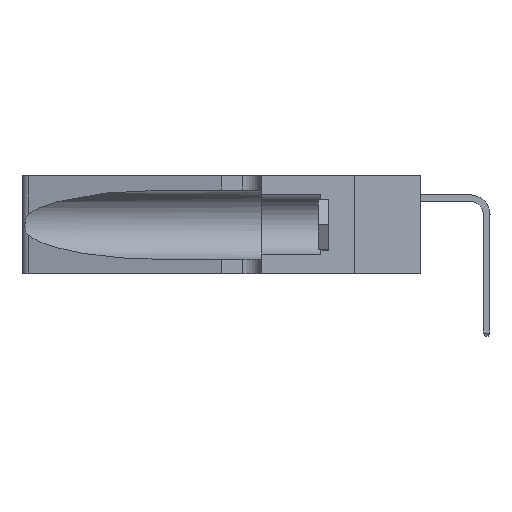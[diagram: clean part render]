
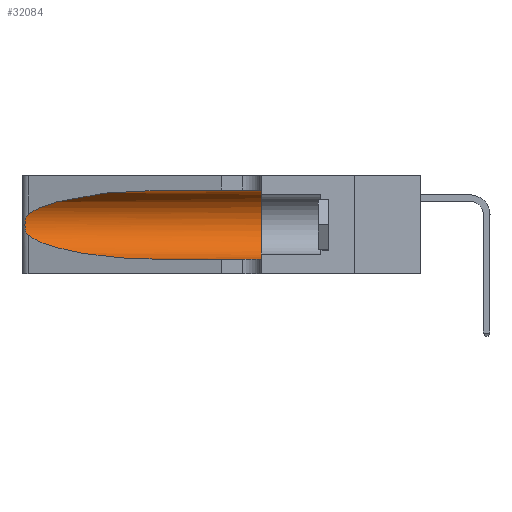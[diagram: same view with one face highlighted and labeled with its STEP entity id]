
A CAD part, left-side view. The second image highlights one B-rep face of the part: STEP entity #32084.
In plain terms, the highlighted cylindrical face has radius 3.308 mm (diameter 6.617 mm), a partial arc.
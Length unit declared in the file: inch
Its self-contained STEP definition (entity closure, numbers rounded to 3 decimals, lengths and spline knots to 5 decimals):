
#2858 = LINE ( 'NONE', #45929, #22922 ) ;
#3886 = CARTESIAN_POINT ( 'NONE',  ( 0.25787, 1.23484, 0.2124 ) ) ;
#4280 = ORIENTED_EDGE ( 'NONE', *, *, #10704, .T. ) ;
#4715 = CARTESIAN_POINT ( 'NONE',  ( 0.1305, 0.35, 0.05475 ) ) ;
#7629 = CARTESIAN_POINT ( 'NONE',  ( 0.26018, 1.23835, 0.19895 ) ) ;
#7790 = LINE ( 'NONE', #32172, #27895 ) ;
#8375 =( BOUNDED_CURVE ( )  B_SPLINE_CURVE ( 3, ( #46101, #42348, #19927, #23691 ),
 .UNSPECIFIED., .F., .F. ) 
 B_SPLINE_CURVE_WITH_KNOTS ( ( 4, 4 ),
 ( 1.5708, 2.84003 ),
 .UNSPECIFIED. ) 
 CURVE ( )  GEOMETRIC_REPRESENTATION_ITEM ( )  RATIONAL_B_SPLINE_CURVE ( ( 1., 0.87, 0.87, 1. ) ) 
 REPRESENTATION_ITEM ( '' )  );
#9575 = DIRECTION ( 'NONE',  ( 0., -1., 0. ) ) ;
#10704 = EDGE_CURVE ( 'NONE', #14904, #12338, #38522, .T. ) ;
#11465 = CARTESIAN_POINT ( 'NONE',  ( 0.26075, 1.23896, 0.178 ) ) ;
#12136 = EDGE_CURVE ( 'NONE', #32609, #28590, #2858, .T. ) ;
#12164 = EDGE_CURVE ( 'NONE', #32609, #22208, #8375, .T. ) ;
#12338 = VERTEX_POINT ( 'NONE', #47231 ) ;
#13855 = B_SPLINE_CURVE_WITH_KNOTS ( 'NONE', 3,
 ( #45111, #18906, #26467, #3886, #30233, #7629, #33977, #11465, #37732, #15300, #41510, #19059, #45274, #22856 ),
 .UNSPECIFIED., .F., .F.,
 ( 4, 2, 2, 2, 2, 2, 4 ),
 ( 0., 0.00027, 0.00053, 0.00107, 0.0016, 0.00187, 0.00214 ),
 .UNSPECIFIED. ) ;
#13954 = DIRECTION ( 'NONE',  ( 0., 0., -1. ) ) ;
#14749 = CARTESIAN_POINT ( 'NONE',  ( 0.18966, 0.96281, 0.05475 ) ) ;
#14904 = VERTEX_POINT ( 'NONE', #39498 ) ;
#15300 = CARTESIAN_POINT ( 'NONE',  ( 0.25856, 1.23593, 0.16098 ) ) ;
#16971 = EDGE_CURVE ( 'NONE', #28590, #46605, #36760, .T. ) ;
#18906 = CARTESIAN_POINT ( 'NONE',  ( 0.25555, 1.22994, 0.2215 ) ) ;
#19059 = CARTESIAN_POINT ( 'NONE',  ( 0.25639, 1.23186, 0.15144 ) ) ;
#19927 = CARTESIAN_POINT ( 'NONE',  ( 0.2373, 1.15595, 0.28018 ) ) ;
#21382 = CARTESIAN_POINT ( 'NONE',  ( 0.1305, 0.35, 0.31525 ) ) ;
#21404 = DIRECTION ( 'NONE',  ( 0., 1., 0. ) ) ;
#22028 = CYLINDRICAL_SURFACE ( 'NONE', #26844, 0.13025 ) ;
#22208 = VERTEX_POINT ( 'NONE', #44135 ) ;
#22330 = CARTESIAN_POINT ( 'NONE',  ( 0.25487, 1.22718, 0.14631 ) ) ;
#22856 = CARTESIAN_POINT ( 'NONE',  ( 0.25487, 1.22718, 0.14631 ) ) ;
#22922 = VECTOR ( 'NONE', #38398, 39.37008 ) ;
#23357 = ORIENTED_EDGE ( 'NONE', *, *, #12136, .F. ) ;
#23691 = CARTESIAN_POINT ( 'NONE',  ( 0.25487, 1.22718, 0.22369 ) ) ;
#26467 = CARTESIAN_POINT ( 'NONE',  ( 0.25639, 1.23184, 0.21858 ) ) ;
#26844 = AXIS2_PLACEMENT_3D ( 'NONE', #28940, #40171, #13954 ) ;
#26999 = ORIENTED_EDGE ( 'NONE', *, *, #12164, .T. ) ;
#27895 = VECTOR ( 'NONE', #9575, 39.37008 ) ;
#28590 = VERTEX_POINT ( 'NONE', #21382 ) ;
#28940 = CARTESIAN_POINT ( 'NONE',  ( 0.1305, 1.61858, 0.185 ) ) ;
#30233 = CARTESIAN_POINT ( 'NONE',  ( 0.25854, 1.2359, 0.20912 ) ) ;
#32084 = ADVANCED_FACE ( 'NONE', ( #41922 ), #22028, .F. ) ;
#32172 = CARTESIAN_POINT ( 'NONE',  ( 0.1305, 1.61858, 0.05475 ) ) ;
#32609 = VERTEX_POINT ( 'NONE', #36390 ) ;
#32693 = EDGE_LOOP ( 'NONE', ( #26999, #33286, #4280, #45901, #33306, #23357 ) ) ;
#33286 = ORIENTED_EDGE ( 'NONE', *, *, #44999, .T. ) ;
#33306 = ORIENTED_EDGE ( 'NONE', *, *, #16971, .F. ) ;
#33977 = CARTESIAN_POINT ( 'NONE',  ( 0.26075, 1.23896, 0.19203 ) ) ;
#36145 = AXIS2_PLACEMENT_3D ( 'NONE', #43827, #21404, #47603 ) ;
#36390 = CARTESIAN_POINT ( 'NONE',  ( 0.1305, 0.72297, 0.31525 ) ) ;
#36760 = CIRCLE ( 'NONE', #36145, 0.13025 ) ;
#37732 = CARTESIAN_POINT ( 'NONE',  ( 0.26017, 1.23833, 0.17102 ) ) ;
#38398 = DIRECTION ( 'NONE',  ( 0., -1., 0. ) ) ;
#38522 =( BOUNDED_CURVE ( )  B_SPLINE_CURVE ( 3, ( #22330, #40964, #14749, #48524 ),
 .UNSPECIFIED., .F., .T. ) 
 B_SPLINE_CURVE_WITH_KNOTS ( ( 4, 4 ),
 ( 3.44316, 4.71239 ),
 .UNSPECIFIED. ) 
 CURVE ( )  GEOMETRIC_REPRESENTATION_ITEM ( )  RATIONAL_B_SPLINE_CURVE ( ( 1., 0.87, 0.87, 1. ) ) 
 REPRESENTATION_ITEM ( '' )  );
#39384 = EDGE_CURVE ( 'NONE', #12338, #46605, #7790, .T. ) ;
#39498 = CARTESIAN_POINT ( 'NONE',  ( 0.25487, 1.22718, 0.14631 ) ) ;
#40171 = DIRECTION ( 'NONE',  ( 0., -1., 0. ) ) ;
#40964 = CARTESIAN_POINT ( 'NONE',  ( 0.2373, 1.15595, 0.08982 ) ) ;
#41510 = CARTESIAN_POINT ( 'NONE',  ( 0.25789, 1.23486, 0.15765 ) ) ;
#41922 = FACE_OUTER_BOUND ( 'NONE', #32693, .T. ) ;
#42348 = CARTESIAN_POINT ( 'NONE',  ( 0.18966, 0.96281, 0.31525 ) ) ;
#43827 = CARTESIAN_POINT ( 'NONE',  ( 0.1305, 0.35, 0.185 ) ) ;
#44135 = CARTESIAN_POINT ( 'NONE',  ( 0.25487, 1.22718, 0.22369 ) ) ;
#44999 = EDGE_CURVE ( 'NONE', #22208, #14904, #13855, .T. ) ;
#45111 = CARTESIAN_POINT ( 'NONE',  ( 0.25487, 1.22718, 0.22369 ) ) ;
#45274 = CARTESIAN_POINT ( 'NONE',  ( 0.25555, 1.22993, 0.14849 ) ) ;
#45901 = ORIENTED_EDGE ( 'NONE', *, *, #39384, .T. ) ;
#45929 = CARTESIAN_POINT ( 'NONE',  ( 0.1305, 1.61858, 0.31525 ) ) ;
#46101 = CARTESIAN_POINT ( 'NONE',  ( 0.1305, 0.72297, 0.31525 ) ) ;
#46605 = VERTEX_POINT ( 'NONE', #4715 ) ;
#47231 = CARTESIAN_POINT ( 'NONE',  ( 0.1305, 0.72297, 0.05475 ) ) ;
#47603 = DIRECTION ( 'NONE',  ( 0., 0., 1. ) ) ;
#48524 = CARTESIAN_POINT ( 'NONE',  ( 0.1305, 0.72297, 0.05475 ) ) ;
